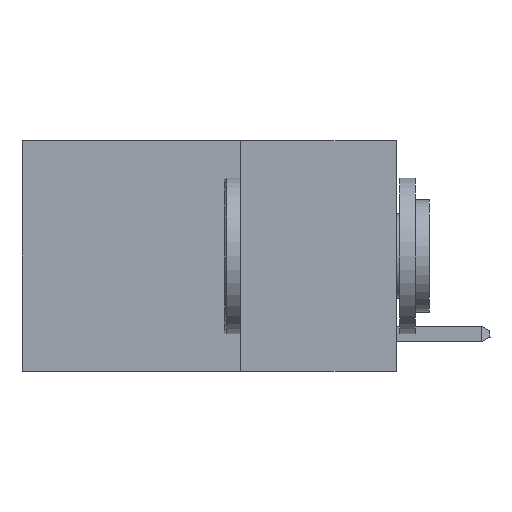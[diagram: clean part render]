
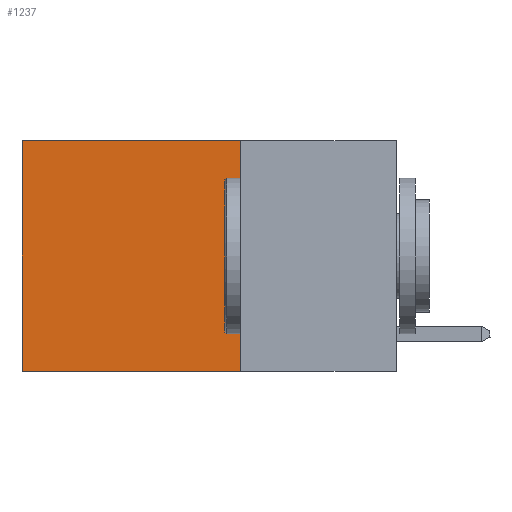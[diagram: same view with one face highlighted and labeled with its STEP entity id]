
A CAD part, left-side view. The second image highlights one B-rep face of the part: STEP entity #1237.
In plain terms, the highlighted planar face has unit normal (-1, 0, 0).
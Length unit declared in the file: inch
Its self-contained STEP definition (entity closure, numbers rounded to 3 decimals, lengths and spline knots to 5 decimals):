
#175 = FACE_OUTER_BOUND ( 'NONE', #11143, .T. ) ;
#293 = CARTESIAN_POINT ( 'NONE',  ( 0.2625, 0.25, 0. ) ) ;
#412 = EDGE_CURVE ( 'NONE', #7411, #10267, #3736, .T. ) ;
#935 = ORIENTED_EDGE ( 'NONE', *, *, #412, .T. ) ;
#1237 = ADVANCED_FACE ( 'NONE', ( #175 ), #11161, .F. ) ;
#2303 = EDGE_CURVE ( 'NONE', #11354, #7411, #2859, .T. ) ;
#2702 = EDGE_CURVE ( 'NONE', #9664, #10267, #10551, .T. ) ;
#2826 = LINE ( 'NONE', #7287, #10213 ) ;
#2859 = LINE ( 'NONE', #3571, #5905 ) ;
#3571 = CARTESIAN_POINT ( 'NONE',  ( 0.2625, 0.25, 0. ) ) ;
#3736 = LINE ( 'NONE', #7415, #10941 ) ;
#4220 = AXIS2_PLACEMENT_3D ( 'NONE', #293, #4861, #5794 ) ;
#4861 = DIRECTION ( 'NONE',  ( 1., 0., 0. ) ) ;
#5193 = CARTESIAN_POINT ( 'NONE',  ( 0.2625, 0.6, -0.37 ) ) ;
#5234 = CARTESIAN_POINT ( 'NONE',  ( 0.2625, 0.25, -0.37 ) ) ;
#5370 = CARTESIAN_POINT ( 'NONE',  ( 0.2625, 0.25, -0.37 ) ) ;
#5794 = DIRECTION ( 'NONE',  ( 0., 0., -1. ) ) ;
#5851 = DIRECTION ( 'NONE',  ( 0., 0., -1. ) ) ;
#5905 = VECTOR ( 'NONE', #8038, 39.37008 ) ;
#6215 = EDGE_CURVE ( 'NONE', #11354, #9664, #2826, .T. ) ;
#7287 = CARTESIAN_POINT ( 'NONE',  ( 0.2625, 0.25, 0. ) ) ;
#7358 = CARTESIAN_POINT ( 'NONE',  ( 0.2625, 0.6, 0. ) ) ;
#7411 = VERTEX_POINT ( 'NONE', #7358 ) ;
#7415 = CARTESIAN_POINT ( 'NONE',  ( 0.2625, 0.6, 0. ) ) ;
#7852 = VECTOR ( 'NONE', #8882, 39.37008 ) ;
#8038 = DIRECTION ( 'NONE',  ( 0., 1., 0. ) ) ;
#8259 = ORIENTED_EDGE ( 'NONE', *, *, #2303, .T. ) ;
#8724 = ORIENTED_EDGE ( 'NONE', *, *, #2702, .F. ) ;
#8882 = DIRECTION ( 'NONE',  ( 0., 1., 0. ) ) ;
#9664 = VERTEX_POINT ( 'NONE', #5370 ) ;
#10071 = CARTESIAN_POINT ( 'NONE',  ( 0.2625, 0.25, 0. ) ) ;
#10213 = VECTOR ( 'NONE', #11097, 39.37008 ) ;
#10267 = VERTEX_POINT ( 'NONE', #5193 ) ;
#10551 = LINE ( 'NONE', #5234, #7852 ) ;
#10941 = VECTOR ( 'NONE', #5851, 39.37008 ) ;
#11097 = DIRECTION ( 'NONE',  ( 0., 0., -1. ) ) ;
#11143 = EDGE_LOOP ( 'NONE', ( #935, #8724, #11220, #8259 ) ) ;
#11161 = PLANE ( 'NONE',  #4220 ) ;
#11220 = ORIENTED_EDGE ( 'NONE', *, *, #6215, .F. ) ;
#11354 = VERTEX_POINT ( 'NONE', #10071 ) ;
